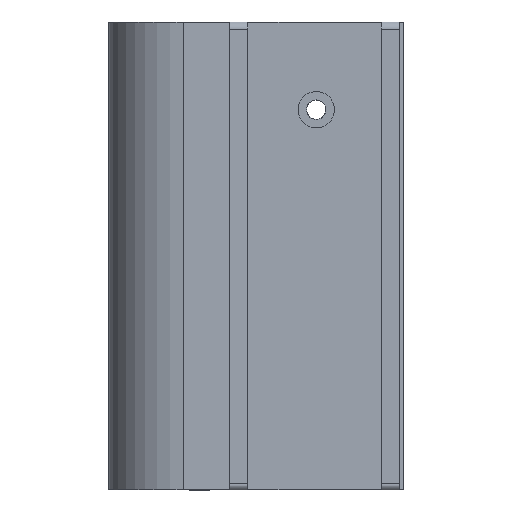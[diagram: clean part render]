
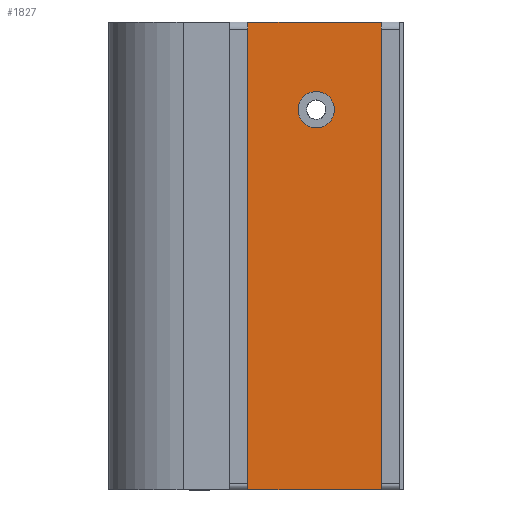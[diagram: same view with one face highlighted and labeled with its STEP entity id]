
A CAD part, left-side view. The second image highlights one B-rep face of the part: STEP entity #1827.
In plain terms, the highlighted planar face has unit normal (-1, 0, 0).
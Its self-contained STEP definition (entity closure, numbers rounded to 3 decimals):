
#49=PLANE('',#1979);
#88=FACE_BOUND('',#247,.T.);
#145=FACE_OUTER_BOUND('',#246,.T.);
#246=EDGE_LOOP('',(#1531,#1532,#1533,#1534));
#247=EDGE_LOOP('',(#1535));
#343=LINE('',#2757,#546);
#445=LINE('',#3009,#648);
#461=LINE('',#3047,#664);
#462=LINE('',#3048,#665);
#546=VECTOR('',#2132,10.);
#648=VECTOR('',#2344,1000.);
#664=VECTOR('',#2388,1000.);
#665=VECTOR('',#2389,10.);
#749=CIRCLE('',#1980,3.);
#813=VERTEX_POINT('',#2754);
#814=VERTEX_POINT('',#2756);
#908=VERTEX_POINT('',#3006);
#909=VERTEX_POINT('',#3008);
#918=VERTEX_POINT('',#3049);
#998=EDGE_CURVE('',#813,#814,#343,.T.);
#1127=EDGE_CURVE('',#908,#909,#445,.T.);
#1147=EDGE_CURVE('',#909,#813,#461,.T.);
#1148=EDGE_CURVE('',#908,#814,#462,.T.);
#1149=EDGE_CURVE('',#918,#918,#749,.T.);
#1531=ORIENTED_EDGE('',*,*,#1147,.F.);
#1532=ORIENTED_EDGE('',*,*,#1127,.F.);
#1533=ORIENTED_EDGE('',*,*,#1148,.T.);
#1534=ORIENTED_EDGE('',*,*,#998,.F.);
#1535=ORIENTED_EDGE('',*,*,#1149,.T.);
#1827=ADVANCED_FACE('',(#145,#88),#49,.T.);
#1979=AXIS2_PLACEMENT_3D('',#3046,#2386,#2387);
#1980=AXIS2_PLACEMENT_3D('',#3050,#2390,#2391);
#2132=DIRECTION('',(0.,-1.,0.));
#2344=DIRECTION('',(0.,1.,0.));
#2386=DIRECTION('center_axis',(-1.,0.,0.));
#2387=DIRECTION('ref_axis',(0.,0.,
1.));
#2388=DIRECTION('',(0.,0.,1.));
#2389=DIRECTION('',(0.,0.,1.));
#2390=DIRECTION('center_axis',(1.,0.,0.));
#2391=DIRECTION('ref_axis',(0.,0.,-1.));
#2754=CARTESIAN_POINT('',(-13.,15.,76.189));
#2756=CARTESIAN_POINT('',(-13.,-7.,76.189));
#2757=CARTESIAN_POINT('',(-13.,-9.122,76.189));
#3006=CARTESIAN_POINT('',(-13.,-7.,-1.));
#3008=CARTESIAN_POINT('',(-13.,15.,-1.));
#3009=CARTESIAN_POINT('',(-13.,-5.,-1.));
#3046=CARTESIAN_POINT('Origin',(-13.,-10.668,-1.));
#3047=CARTESIAN_POINT('',(-13.,15.,-1.));
#3048=CARTESIAN_POINT('',(-13.,-7.,18.297));
#3049=CARTESIAN_POINT('',(-13.,3.736,64.727));
#3050=CARTESIAN_POINT('Origin',(-13.,3.736,61.727));
